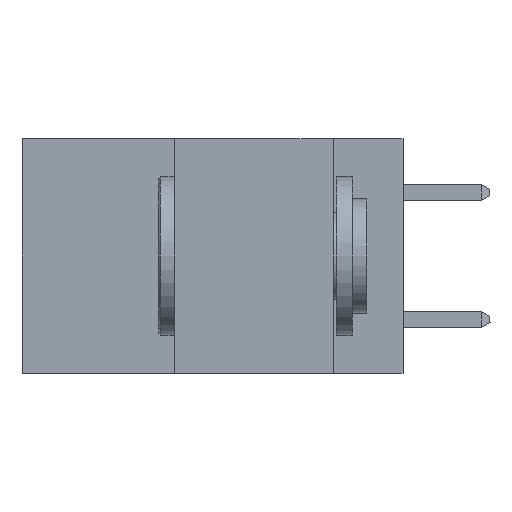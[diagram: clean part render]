
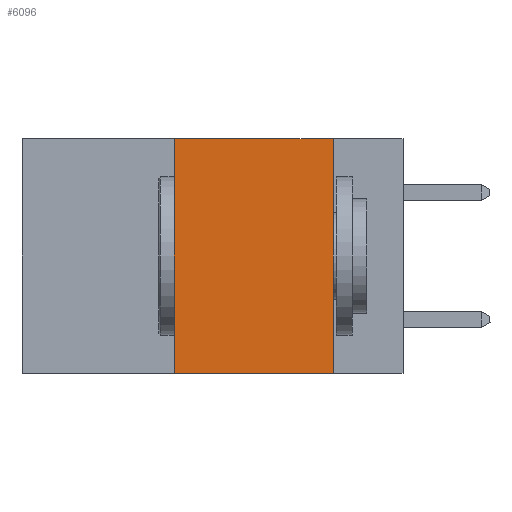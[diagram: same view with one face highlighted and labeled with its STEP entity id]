
A CAD part, left-side view. The second image highlights one B-rep face of the part: STEP entity #6096.
In plain terms, the highlighted planar face has unit normal (-1, 0, 0).
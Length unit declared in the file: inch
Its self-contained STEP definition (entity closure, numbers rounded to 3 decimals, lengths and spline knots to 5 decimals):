
#1508 = ORIENTED_EDGE ( 'NONE', *, *, #19993, .F. ) ;
#3015 = VECTOR ( 'NONE', #23175, 39.37008 ) ;
#4968 = EDGE_CURVE ( 'NONE', #40155, #10140, #12185, .T. ) ;
#5421 = EDGE_LOOP ( 'NONE', ( #1508, #18151, #32431, #29389 ) ) ;
#5563 = DIRECTION ( 'NONE',  ( 0., 0., -1. ) ) ;
#6096 = ADVANCED_FACE ( 'NONE', ( #35678 ), #22216, .F. ) ;
#6447 = CARTESIAN_POINT ( 'NONE',  ( 0., 0.6, 0. ) ) ;
#7864 = DIRECTION ( 'NONE',  ( 0., -1., 0. ) ) ;
#10140 = VERTEX_POINT ( 'NONE', #14840 ) ;
#12185 = LINE ( 'NONE', #16729, #3015 ) ;
#12246 = DIRECTION ( 'NONE',  ( 1., 0., 0. ) ) ;
#12750 = LINE ( 'NONE', #14600, #38841 ) ;
#14600 = CARTESIAN_POINT ( 'NONE',  ( 0., 0.11, 0. ) ) ;
#14840 = CARTESIAN_POINT ( 'NONE',  ( 0., 0.36, 0. ) ) ;
#16729 = CARTESIAN_POINT ( 'NONE',  ( 0., 0.36, 0. ) ) ;
#17254 = VECTOR ( 'NONE', #20195, 39.37008 ) ;
#18151 = ORIENTED_EDGE ( 'NONE', *, *, #29602, .F. ) ;
#19345 = LINE ( 'NONE', #6447, #36754 ) ;
#19993 = EDGE_CURVE ( 'NONE', #33901, #24475, #12750, .T. ) ;
#20195 = DIRECTION ( 'NONE',  ( 0., -1., 0. ) ) ;
#21652 = AXIS2_PLACEMENT_3D ( 'NONE', #38688, #12246, #5563 ) ;
#22216 = PLANE ( 'NONE',  #21652 ) ;
#23175 = DIRECTION ( 'NONE',  ( 0., 0., 1. ) ) ;
#24475 = VERTEX_POINT ( 'NONE', #37075 ) ;
#29389 = ORIENTED_EDGE ( 'NONE', *, *, #36953, .T. ) ;
#29602 = EDGE_CURVE ( 'NONE', #10140, #33901, #19345, .T. ) ;
#30634 = CARTESIAN_POINT ( 'NONE',  ( 0., 0.11, 0. ) ) ;
#31610 = CARTESIAN_POINT ( 'NONE',  ( 0., 0.36, -0.37 ) ) ;
#32431 = ORIENTED_EDGE ( 'NONE', *, *, #4968, .F. ) ;
#33153 = LINE ( 'NONE', #33230, #17254 ) ;
#33230 = CARTESIAN_POINT ( 'NONE',  ( 0., 0.6, -0.37 ) ) ;
#33901 = VERTEX_POINT ( 'NONE', #30634 ) ;
#35678 = FACE_OUTER_BOUND ( 'NONE', #5421, .T. ) ;
#36754 = VECTOR ( 'NONE', #7864, 39.37008 ) ;
#36953 = EDGE_CURVE ( 'NONE', #40155, #24475, #33153, .T. ) ;
#37075 = CARTESIAN_POINT ( 'NONE',  ( 0., 0.11, -0.37 ) ) ;
#38688 = CARTESIAN_POINT ( 'NONE',  ( 0., 0.6, 0. ) ) ;
#38841 = VECTOR ( 'NONE', #40749, 39.37008 ) ;
#40155 = VERTEX_POINT ( 'NONE', #31610 ) ;
#40749 = DIRECTION ( 'NONE',  ( 0., 0., -1. ) ) ;
